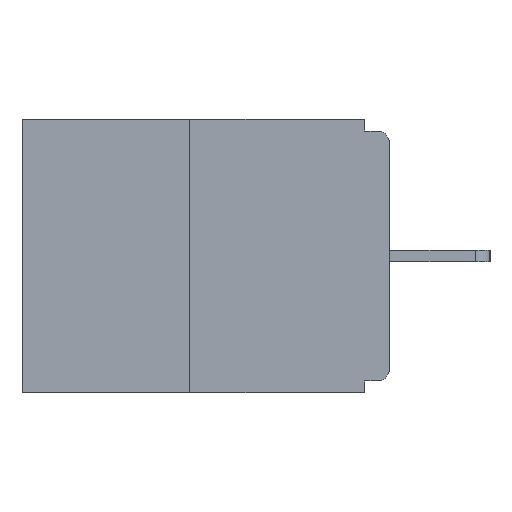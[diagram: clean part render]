
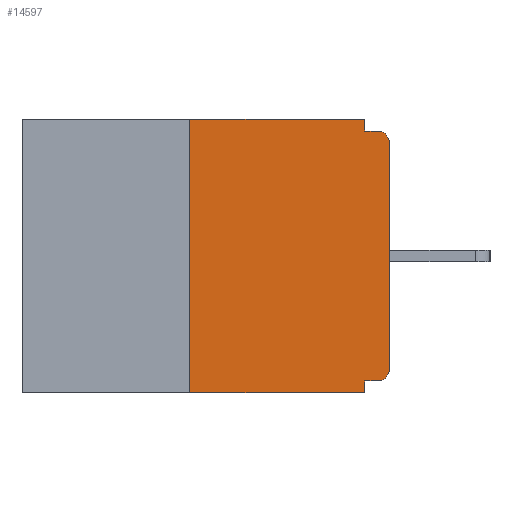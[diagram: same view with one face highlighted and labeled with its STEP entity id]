
A CAD part, left-side view. The second image highlights one B-rep face of the part: STEP entity #14597.
In plain terms, the highlighted planar face has unit normal (-1, 0, 0).
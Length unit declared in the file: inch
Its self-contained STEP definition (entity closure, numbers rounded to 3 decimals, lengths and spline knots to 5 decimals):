
#72 = DIRECTION ( 'NONE',  ( 0., 0., 1. ) ) ;
#624 = EDGE_CURVE ( 'NONE', #7444, #23072, #15795, .T. ) ;
#882 = AXIS2_PLACEMENT_3D ( 'NONE', #2641, #23045, #4812 ) ;
#1069 = CARTESIAN_POINT ( 'NONE',  ( 0., 0., -0.328 ) ) ;
#1497 = ORIENTED_EDGE ( 'NONE', *, *, #23048, .F. ) ;
#1533 = CARTESIAN_POINT ( 'NONE',  ( 0., 0.015, -0.015 ) ) ;
#1601 = VERTEX_POINT ( 'NONE', #20460 ) ;
#1641 = ORIENTED_EDGE ( 'NONE', *, *, #8232, .T. ) ;
#1970 = LINE ( 'NONE', #24921, #2313 ) ;
#2313 = VECTOR ( 'NONE', #72, 39.37008 ) ;
#2640 = ORIENTED_EDGE ( 'NONE', *, *, #13268, .T. ) ;
#2641 = CARTESIAN_POINT ( 'NONE',  ( 0., 0.015, -0.313 ) ) ;
#2648 = CARTESIAN_POINT ( 'NONE',  ( 0., 0.46, 0. ) ) ;
#2803 = CARTESIAN_POINT ( 'NONE',  ( 0., 0.46, -0.343 ) ) ;
#2976 = CARTESIAN_POINT ( 'NONE',  ( 0., 0.25, -0.343 ) ) ;
#3629 = VECTOR ( 'NONE', #25295, 39.37008 ) ;
#4407 = DIRECTION ( 'NONE',  ( 1., 0., 0. ) ) ;
#4812 = DIRECTION ( 'NONE',  ( 0., 0., -1. ) ) ;
#4882 = CARTESIAN_POINT ( 'NONE',  ( 0., 0., -0.015 ) ) ;
#5260 = EDGE_CURVE ( 'NONE', #12544, #8682, #9870, .T. ) ;
#6456 = LINE ( 'NONE', #2803, #12998 ) ;
#6594 = AXIS2_PLACEMENT_3D ( 'NONE', #12759, #16949, #14642 ) ;
#6759 = VERTEX_POINT ( 'NONE', #12319 ) ;
#7444 = VERTEX_POINT ( 'NONE', #24010 ) ;
#7914 = VECTOR ( 'NONE', #19859, 39.37008 ) ;
#8114 = ORIENTED_EDGE ( 'NONE', *, *, #5260, .F. ) ;
#8232 = EDGE_CURVE ( 'NONE', #22848, #6759, #11400, .T. ) ;
#8682 = VERTEX_POINT ( 'NONE', #21680 ) ;
#8877 = VERTEX_POINT ( 'NONE', #13005 ) ;
#9657 = VECTOR ( 'NONE', #23546, 39.37008 ) ;
#9870 = LINE ( 'NONE', #11783, #15182 ) ;
#10664 = VECTOR ( 'NONE', #19650, 39.37008 ) ;
#10767 = ORIENTED_EDGE ( 'NONE', *, *, #23791, .T. ) ;
#11014 = LINE ( 'NONE', #12896, #3629 ) ;
#11400 = LINE ( 'NONE', #21806, #10664 ) ;
#11613 = LINE ( 'NONE', #1069, #7914 ) ;
#11783 = CARTESIAN_POINT ( 'NONE',  ( 0., 0.46, 0. ) ) ;
#12134 = EDGE_LOOP ( 'NONE', ( #8114, #14041, #19021, #20846, #1497, #2640, #1641, #10767, #20778, #24667 ) ) ;
#12319 = CARTESIAN_POINT ( 'NONE',  ( 0., 0., -0.03 ) ) ;
#12544 = VERTEX_POINT ( 'NONE', #12967 ) ;
#12759 = CARTESIAN_POINT ( 'NONE',  ( 0., 0.015, -0.03 ) ) ;
#12896 = CARTESIAN_POINT ( 'NONE',  ( 0., 0.031, 0. ) ) ;
#12967 = CARTESIAN_POINT ( 'NONE',  ( 0., 0.25, 0. ) ) ;
#12998 = VECTOR ( 'NONE', #25071, 39.37008 ) ;
#13005 = CARTESIAN_POINT ( 'NONE',  ( 0., 0.031, -0.015 ) ) ;
#13268 = EDGE_CURVE ( 'NONE', #1601, #22848, #14706, .T. ) ;
#14041 = ORIENTED_EDGE ( 'NONE', *, *, #17810, .F. ) ;
#14597 = ADVANCED_FACE ( 'NONE', ( #24912 ), #16980, .F. ) ;
#14642 = DIRECTION ( 'NONE',  ( 0., 0., -1. ) ) ;
#14706 = CIRCLE ( 'NONE', #882, 0.015 ) ;
#15138 = DIRECTION ( 'NONE',  ( 0., -1., 0. ) ) ;
#15182 = VECTOR ( 'NONE', #24327, 39.37008 ) ;
#15540 = LINE ( 'NONE', #4882, #23002 ) ;
#15795 = LINE ( 'NONE', #24009, #9657 ) ;
#16909 = CARTESIAN_POINT ( 'NONE',  ( 0., 0., -0.313 ) ) ;
#16949 = DIRECTION ( 'NONE',  ( -1., 0., 0. ) ) ;
#16980 = PLANE ( 'NONE',  #22071 ) ;
#17390 = CIRCLE ( 'NONE', #6594, 0.015 ) ;
#17745 = VERTEX_POINT ( 'NONE', #2976 ) ;
#17810 = EDGE_CURVE ( 'NONE', #17745, #12544, #1970, .T. ) ;
#18430 = EDGE_CURVE ( 'NONE', #8682, #8877, #11014, .T. ) ;
#19021 = ORIENTED_EDGE ( 'NONE', *, *, #20499, .T. ) ;
#19650 = DIRECTION ( 'NONE',  ( 0., 0., 1. ) ) ;
#19859 = DIRECTION ( 'NONE',  ( 0., 1., 0. ) ) ;
#20460 = CARTESIAN_POINT ( 'NONE',  ( 0., 0.015, -0.328 ) ) ;
#20499 = EDGE_CURVE ( 'NONE', #17745, #23072, #6456, .T. ) ;
#20778 = ORIENTED_EDGE ( 'NONE', *, *, #23070, .F. ) ;
#20846 = ORIENTED_EDGE ( 'NONE', *, *, #624, .F. ) ;
#21024 = DIRECTION ( 'NONE',  ( 0., 0., -1. ) ) ;
#21680 = CARTESIAN_POINT ( 'NONE',  ( 0., 0.031, 0. ) ) ;
#21806 = CARTESIAN_POINT ( 'NONE',  ( 0., 0., 0. ) ) ;
#22071 = AXIS2_PLACEMENT_3D ( 'NONE', #2648, #4407, #21024 ) ;
#22453 = VERTEX_POINT ( 'NONE', #1533 ) ;
#22848 = VERTEX_POINT ( 'NONE', #16909 ) ;
#23002 = VECTOR ( 'NONE', #15138, 39.37008 ) ;
#23045 = DIRECTION ( 'NONE',  ( -1., 0., 0. ) ) ;
#23048 = EDGE_CURVE ( 'NONE', #1601, #7444, #11613, .T. ) ;
#23070 = EDGE_CURVE ( 'NONE', #8877, #22453, #15540, .T. ) ;
#23072 = VERTEX_POINT ( 'NONE', #23772 ) ;
#23546 = DIRECTION ( 'NONE',  ( 0., 0., -1. ) ) ;
#23772 = CARTESIAN_POINT ( 'NONE',  ( 0., 0.031, -0.343 ) ) ;
#23791 = EDGE_CURVE ( 'NONE', #6759, #22453, #17390, .T. ) ;
#24009 = CARTESIAN_POINT ( 'NONE',  ( 0., 0.031, -0.343 ) ) ;
#24010 = CARTESIAN_POINT ( 'NONE',  ( 0., 0.031, -0.328 ) ) ;
#24327 = DIRECTION ( 'NONE',  ( 0., -1., 0. ) ) ;
#24667 = ORIENTED_EDGE ( 'NONE', *, *, #18430, .F. ) ;
#24912 = FACE_OUTER_BOUND ( 'NONE', #12134, .T. ) ;
#24921 = CARTESIAN_POINT ( 'NONE',  ( 0., 0.25, 0. ) ) ;
#25071 = DIRECTION ( 'NONE',  ( 0., -1., 0. ) ) ;
#25295 = DIRECTION ( 'NONE',  ( 0., 0., -1. ) ) ;
